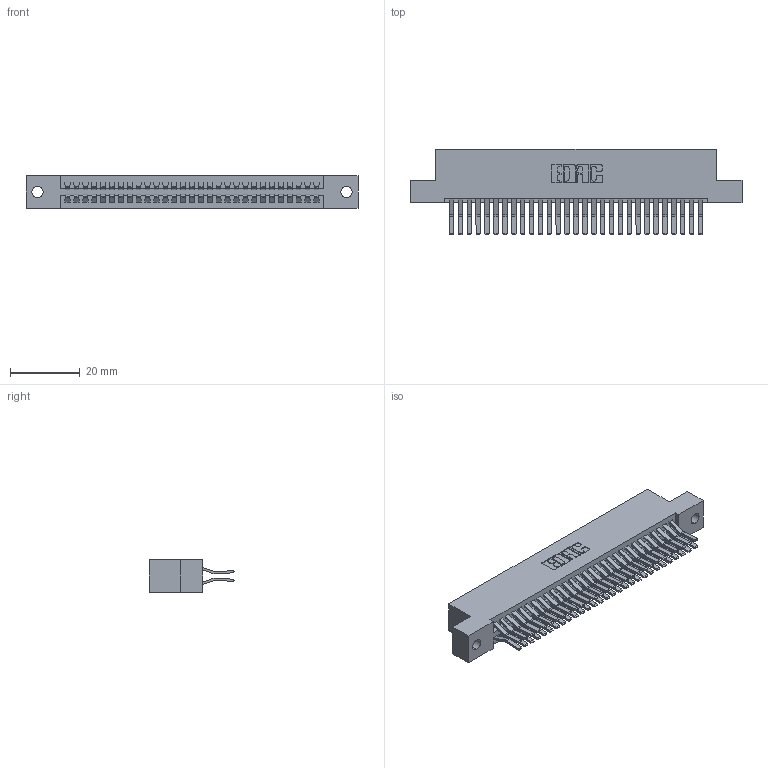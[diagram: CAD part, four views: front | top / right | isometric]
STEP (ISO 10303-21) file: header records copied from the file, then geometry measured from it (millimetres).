
FILE_DESCRIPTION (( 'STEP AP203' ), '1' );
FILE_NAME ('345-058-560-202.STEP', '2018-09-26T18:42:56', ( '' ), ( '' ), 'SwSTEP 2.0', 'SolidWorks 2016', '' );
FILE_SCHEMA (( 'CONFIG_CONTROL_DESIGN' ));
Length unit declared in the file: inch
Products named in the file (3): 345 Part_Flush Mounting Lugs - 0.128 Dia; 345-058-560-202; 345-292-001_560 Tail
Assembly tree (59 placements, depth 2):
  345-058-560-202
    345 Part_Flush Mounting Lugs - 0.128 Dia
    345-292-001_560 Tail  x58
Bounding box: 94.87 x 24.45 x 9.4 mm (x, y, z)
Volume: 9438.5 mm3; surface area: 14404.9 mm2
Topology: 59 solids, 59 shells, 3142 faces, 9331 edges, 6142 vertices
Faces by surface type: plane 1994, cylinder 1148
Entity records: 24595 total; most frequent: CARTESIAN_POINT 4136, ORIENTED_EDGE 4070, DIRECTION 3667, EDGE_CURVE 2035, LINE 1783, VECTOR 1783, VERTEX_POINT 1354, AXIS2_PLACEMENT_3D 942
